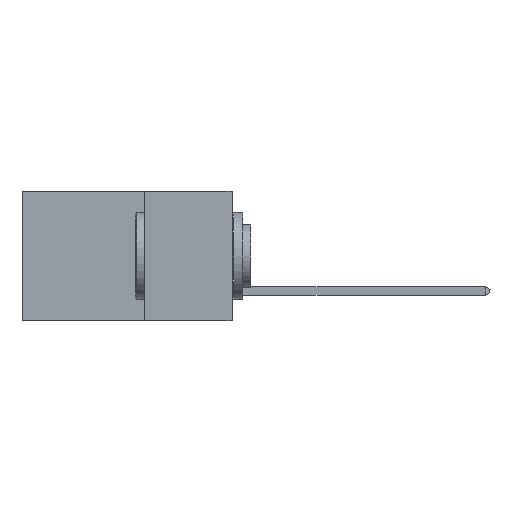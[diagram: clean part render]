
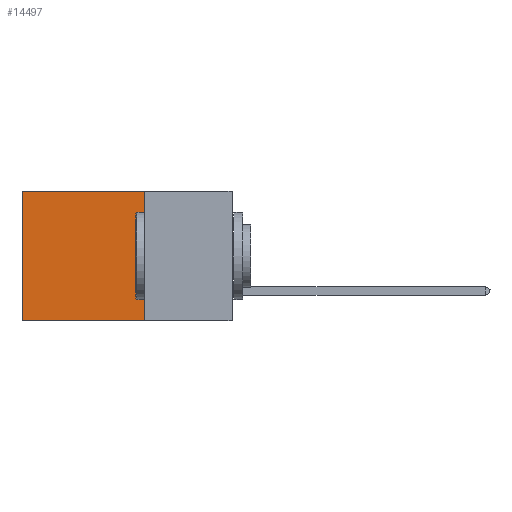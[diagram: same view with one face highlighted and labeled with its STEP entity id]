
A CAD part, left-side view. The second image highlights one B-rep face of the part: STEP entity #14497.
In plain terms, the highlighted planar face has unit normal (-1, 0, 0).
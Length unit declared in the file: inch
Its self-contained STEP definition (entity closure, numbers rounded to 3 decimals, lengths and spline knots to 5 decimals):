
#382 = PLANE ( 'NONE',  #17484 ) ;
#598 = DIRECTION ( 'NONE',  ( 0., 0., -1. ) ) ;
#2016 = DIRECTION ( 'NONE',  ( 0., 0., -1. ) ) ;
#2459 = DIRECTION ( 'NONE',  ( 0., 0., -1. ) ) ;
#2788 = VERTEX_POINT ( 'NONE', #16952 ) ;
#4238 = CARTESIAN_POINT ( 'NONE',  ( 0.2875, 0.25, -0.37 ) ) ;
#4467 = VERTEX_POINT ( 'NONE', #16636 ) ;
#6378 = LINE ( 'NONE', #17734, #10836 ) ;
#7189 = VECTOR ( 'NONE', #2459, 39.37008 ) ;
#8347 = VERTEX_POINT ( 'NONE', #11180 ) ;
#8875 = EDGE_CURVE ( 'NONE', #17273, #2788, #6378, .T. ) ;
#9199 = EDGE_LOOP ( 'NONE', ( #15680, #15757, #15450, #9465 ) ) ;
#9465 = ORIENTED_EDGE ( 'NONE', *, *, #14748, .T. ) ;
#9692 = LINE ( 'NONE', #12273, #14667 ) ;
#10836 = VECTOR ( 'NONE', #16368, 39.37008 ) ;
#11180 = CARTESIAN_POINT ( 'NONE',  ( 0.2875, 0.25, 0. ) ) ;
#11516 = CARTESIAN_POINT ( 'NONE',  ( 0.2875, 0.25, 0. ) ) ;
#11701 = CARTESIAN_POINT ( 'NONE',  ( 0.2875, 0.6, 0. ) ) ;
#12273 = CARTESIAN_POINT ( 'NONE',  ( 0.2875, 0.25, 0. ) ) ;
#14364 = LINE ( 'NONE', #11701, #17150 ) ;
#14497 = ADVANCED_FACE ( 'NONE', ( #16963 ), #382, .F. ) ;
#14667 = VECTOR ( 'NONE', #15354, 39.37008 ) ;
#14748 = EDGE_CURVE ( 'NONE', #8347, #4467, #9692, .T. ) ;
#14999 = CARTESIAN_POINT ( 'NONE',  ( 0.2875, 0.25, 0. ) ) ;
#15354 = DIRECTION ( 'NONE',  ( 0., 1., 0. ) ) ;
#15450 = ORIENTED_EDGE ( 'NONE', *, *, #15759, .F. ) ;
#15680 = ORIENTED_EDGE ( 'NONE', *, *, #16035, .T. ) ;
#15757 = ORIENTED_EDGE ( 'NONE', *, *, #8875, .F. ) ;
#15759 = EDGE_CURVE ( 'NONE', #8347, #17273, #16390, .T. ) ;
#16035 = EDGE_CURVE ( 'NONE', #4467, #2788, #14364, .T. ) ;
#16266 = DIRECTION ( 'NONE',  ( 1., 0., 0. ) ) ;
#16368 = DIRECTION ( 'NONE',  ( 0., 1., 0. ) ) ;
#16390 = LINE ( 'NONE', #14999, #7189 ) ;
#16636 = CARTESIAN_POINT ( 'NONE',  ( 0.2875, 0.6, 0. ) ) ;
#16952 = CARTESIAN_POINT ( 'NONE',  ( 0.2875, 0.6, -0.37 ) ) ;
#16963 = FACE_OUTER_BOUND ( 'NONE', #9199, .T. ) ;
#17150 = VECTOR ( 'NONE', #2016, 39.37008 ) ;
#17273 = VERTEX_POINT ( 'NONE', #4238 ) ;
#17484 = AXIS2_PLACEMENT_3D ( 'NONE', #11516, #16266, #598 ) ;
#17734 = CARTESIAN_POINT ( 'NONE',  ( 0.2875, 0.25, -0.37 ) ) ;
